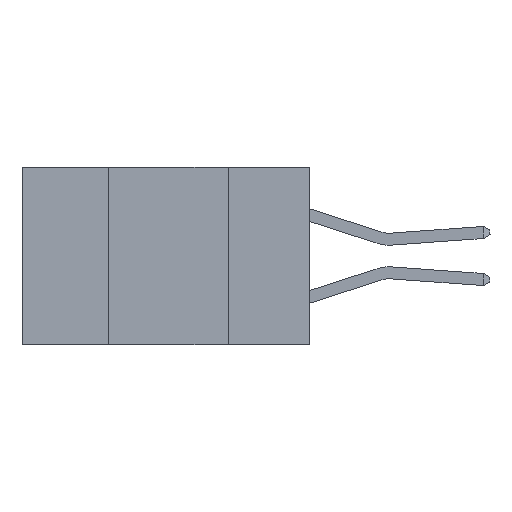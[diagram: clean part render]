
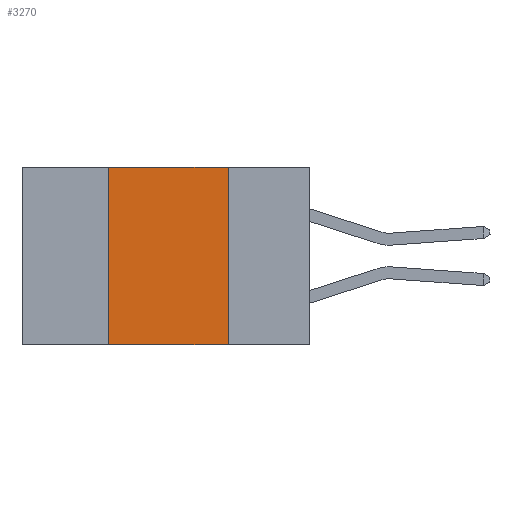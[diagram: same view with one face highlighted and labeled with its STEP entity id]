
A CAD part, left-side view. The second image highlights one B-rep face of the part: STEP entity #3270.
In plain terms, the highlighted planar face has unit normal (-1, 0, 0).
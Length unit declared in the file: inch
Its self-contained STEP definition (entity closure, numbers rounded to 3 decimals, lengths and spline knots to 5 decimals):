
#74 = CARTESIAN_POINT ( 'NONE',  ( 0., 0.42, 0. ) ) ;
#124 = VECTOR ( 'NONE', #4077, 39.37008 ) ;
#673 = ORIENTED_EDGE ( 'NONE', *, *, #6312, .T. ) ;
#1448 = EDGE_CURVE ( 'NONE', #3625, #11688, #2171, .T. ) ;
#1834 = VECTOR ( 'NONE', #11993, 39.37008 ) ;
#2171 = LINE ( 'NONE', #14612, #1834 ) ;
#3270 = ADVANCED_FACE ( 'NONE', ( #9841 ), #12898, .F. ) ;
#3625 = VERTEX_POINT ( 'NONE', #74 ) ;
#4077 = DIRECTION ( 'NONE',  ( 0., 0., 1. ) ) ;
#4117 = DIRECTION ( 'NONE',  ( 0., -1., 0. ) ) ;
#4265 = VERTEX_POINT ( 'NONE', #6625 ) ;
#5965 = CARTESIAN_POINT ( 'NONE',  ( 0., 0.6, -0.37 ) ) ;
#6312 = EDGE_CURVE ( 'NONE', #4265, #6594, #18406, .T. ) ;
#6594 = VERTEX_POINT ( 'NONE', #9765 ) ;
#6625 = CARTESIAN_POINT ( 'NONE',  ( 0., 0.42, -0.37 ) ) ;
#7324 = LINE ( 'NONE', #19722, #15063 ) ;
#8228 = VECTOR ( 'NONE', #4117, 39.37008 ) ;
#8927 = LINE ( 'NONE', #11907, #124 ) ;
#9765 = CARTESIAN_POINT ( 'NONE',  ( 0., 0.17, -0.37 ) ) ;
#9834 = EDGE_CURVE ( 'NONE', #4265, #3625, #8927, .T. ) ;
#9841 = FACE_OUTER_BOUND ( 'NONE', #19202, .T. ) ;
#10660 = EDGE_CURVE ( 'NONE', #11688, #6594, #7324, .T. ) ;
#11688 = VERTEX_POINT ( 'NONE', #19244 ) ;
#11907 = CARTESIAN_POINT ( 'NONE',  ( 0., 0.42, -0.37 ) ) ;
#11993 = DIRECTION ( 'NONE',  ( 0., -1., 0. ) ) ;
#12165 = AXIS2_PLACEMENT_3D ( 'NONE', #17355, #14128, #17269 ) ;
#12898 = PLANE ( 'NONE',  #12165 ) ;
#12899 = ORIENTED_EDGE ( 'NONE', *, *, #1448, .F. ) ;
#14128 = DIRECTION ( 'NONE',  ( 1., 0., 0. ) ) ;
#14484 = ORIENTED_EDGE ( 'NONE', *, *, #9834, .F. ) ;
#14612 = CARTESIAN_POINT ( 'NONE',  ( 0., 0.6, 0. ) ) ;
#14823 = DIRECTION ( 'NONE',  ( 0., 0., -1. ) ) ;
#15063 = VECTOR ( 'NONE', #14823, 39.37008 ) ;
#17269 = DIRECTION ( 'NONE',  ( 0., 0., -1. ) ) ;
#17355 = CARTESIAN_POINT ( 'NONE',  ( 0., 0.6, 0. ) ) ;
#18406 = LINE ( 'NONE', #5965, #8228 ) ;
#19202 = EDGE_LOOP ( 'NONE', ( #19584, #12899, #14484, #673 ) ) ;
#19244 = CARTESIAN_POINT ( 'NONE',  ( 0., 0.17, 0. ) ) ;
#19584 = ORIENTED_EDGE ( 'NONE', *, *, #10660, .F. ) ;
#19722 = CARTESIAN_POINT ( 'NONE',  ( 0., 0.17, -0.37 ) ) ;
